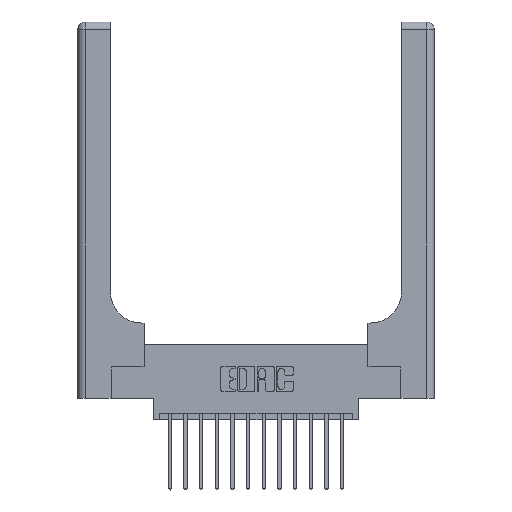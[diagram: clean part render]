
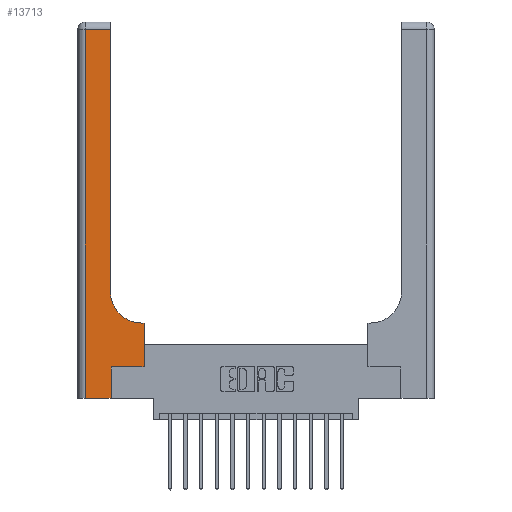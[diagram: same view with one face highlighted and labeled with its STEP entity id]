
A CAD part, top view. The second image highlights one B-rep face of the part: STEP entity #13713.
In plain terms, the highlighted planar face has unit normal (0, 0, 1).
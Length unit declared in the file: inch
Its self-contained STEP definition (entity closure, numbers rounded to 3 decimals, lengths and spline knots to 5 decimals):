
#178 = EDGE_LOOP ( 'NONE', ( #1392, #8823, #4868, #6654, #13039, #760, #14122, #10575, #12890 ) ) ;
#760 = ORIENTED_EDGE ( 'NONE', *, *, #14754, .T. ) ;
#984 = CARTESIAN_POINT ( 'NONE',  ( 0.06, 2.94, 0.37 ) ) ;
#1244 = DIRECTION ( 'NONE',  ( 0., 0., -1. ) ) ;
#1270 = DIRECTION ( 'NONE',  ( 1., 0., 0. ) ) ;
#1392 = ORIENTED_EDGE ( 'NONE', *, *, #10980, .T. ) ;
#1998 = EDGE_CURVE ( 'NONE', #4549, #11544, #16536, .T. ) ;
#2104 = LINE ( 'NONE', #8802, #8312 ) ;
#2680 = DIRECTION ( 'NONE',  ( 0., 0., -1. ) ) ;
#2692 = CARTESIAN_POINT ( 'NONE',  ( 0.26, 2.94, 0.37 ) ) ;
#3514 = EDGE_CURVE ( 'NONE', #14203, #12566, #5330, .T. ) ;
#3596 = VECTOR ( 'NONE', #9896, 39.37008 ) ;
#4549 = VERTEX_POINT ( 'NONE', #10410 ) ;
#4627 = VECTOR ( 'NONE', #4942, 39.37008 ) ;
#4661 = CIRCLE ( 'NONE', #5664, 0.25 ) ;
#4868 = ORIENTED_EDGE ( 'NONE', *, *, #14104, .T. ) ;
#4942 = DIRECTION ( 'NONE',  ( 0., -1., 0. ) ) ;
#5330 = LINE ( 'NONE', #16295, #11973 ) ;
#5664 = AXIS2_PLACEMENT_3D ( 'NONE', #9179, #1244, #10537 ) ;
#5874 = CARTESIAN_POINT ( 'NONE',  ( 0.528, 0.25, 0.37 ) ) ;
#6355 = EDGE_CURVE ( 'NONE', #7479, #15930, #13785, .T. ) ;
#6401 = VERTEX_POINT ( 'NONE', #9953 ) ;
#6654 = ORIENTED_EDGE ( 'NONE', *, *, #6355, .T. ) ;
#7205 = LINE ( 'NONE', #5874, #14267 ) ;
#7479 = VERTEX_POINT ( 'NONE', #8169 ) ;
#7926 = CARTESIAN_POINT ( 'NONE',  ( 0.265, 0., 0.37 ) ) ;
#7965 = CARTESIAN_POINT ( 'NONE',  ( 0., 3., 0.37 ) ) ;
#8169 = CARTESIAN_POINT ( 'NONE',  ( 0.06, 0., 0.37 ) ) ;
#8312 = VECTOR ( 'NONE', #16775, 39.37008 ) ;
#8544 = CARTESIAN_POINT ( 'NONE',  ( 0., 0., 0.37 ) ) ;
#8802 = CARTESIAN_POINT ( 'NONE',  ( 0.265, 0., 0.37 ) ) ;
#8823 = ORIENTED_EDGE ( 'NONE', *, *, #3514, .T. ) ;
#9179 = CARTESIAN_POINT ( 'NONE',  ( 0.51, 0.85, 0.37 ) ) ;
#9453 = VECTOR ( 'NONE', #14989, 39.37008 ) ;
#9690 = DIRECTION ( 'NONE',  ( -1., 0., 0. ) ) ;
#9896 = DIRECTION ( 'NONE',  ( 1., 0., 0. ) ) ;
#9953 = CARTESIAN_POINT ( 'NONE',  ( 0.265, 0.25, 0.37 ) ) ;
#10099 = VECTOR ( 'NONE', #12071, 39.37008 ) ;
#10410 = CARTESIAN_POINT ( 'NONE',  ( 0.528, 0.6, 0.37 ) ) ;
#10510 = LINE ( 'NONE', #10718, #10099 ) ;
#10537 = DIRECTION ( 'NONE',  ( 1., 0., 0. ) ) ;
#10575 = ORIENTED_EDGE ( 'NONE', *, *, #1998, .T. ) ;
#10616 = PLANE ( 'NONE',  #15116 ) ;
#10718 = CARTESIAN_POINT ( 'NONE',  ( 0.26, 3., 0.37 ) ) ;
#10980 = EDGE_CURVE ( 'NONE', #16078, #14203, #10510, .T. ) ;
#11180 = EDGE_CURVE ( 'NONE', #16935, #4549, #7205, .T. ) ;
#11438 = CARTESIAN_POINT ( 'NONE',  ( 0.528, 0.25, 0.37 ) ) ;
#11544 = VERTEX_POINT ( 'NONE', #14835 ) ;
#11868 = LINE ( 'NONE', #17193, #14990 ) ;
#11973 = VECTOR ( 'NONE', #9690, 39.37008 ) ;
#11975 = DIRECTION ( 'NONE',  ( -1., 0., 0. ) ) ;
#12071 = DIRECTION ( 'NONE',  ( 0., 1., 0. ) ) ;
#12566 = VERTEX_POINT ( 'NONE', #984 ) ;
#12890 = ORIENTED_EDGE ( 'NONE', *, *, #13169, .T. ) ;
#12904 = CARTESIAN_POINT ( 'NONE',  ( 0.06, 3., 0.37 ) ) ;
#13039 = ORIENTED_EDGE ( 'NONE', *, *, #15210, .T. ) ;
#13169 = EDGE_CURVE ( 'NONE', #11544, #16078, #4661, .T. ) ;
#13580 = FACE_OUTER_BOUND ( 'NONE', #178, .T. ) ;
#13619 = CARTESIAN_POINT ( 'NONE',  ( 0.26, 0.85, 0.37 ) ) ;
#13666 = CARTESIAN_POINT ( 'NONE',  ( 0.26, 0.6, 0.37 ) ) ;
#13713 = ADVANCED_FACE ( 'NONE', ( #13580 ), #10616, .F. ) ;
#13785 = LINE ( 'NONE', #8544, #3596 ) ;
#13878 = DIRECTION ( 'NONE',  ( 0., 1., 0. ) ) ;
#14104 = EDGE_CURVE ( 'NONE', #12566, #7479, #14810, .T. ) ;
#14122 = ORIENTED_EDGE ( 'NONE', *, *, #11180, .T. ) ;
#14203 = VERTEX_POINT ( 'NONE', #2692 ) ;
#14267 = VECTOR ( 'NONE', #13878, 39.37008 ) ;
#14754 = EDGE_CURVE ( 'NONE', #6401, #16935, #11868, .T. ) ;
#14810 = LINE ( 'NONE', #12904, #4627 ) ;
#14835 = CARTESIAN_POINT ( 'NONE',  ( 0.51, 0.6, 0.37 ) ) ;
#14989 = DIRECTION ( 'NONE',  ( -1., 0., 0. ) ) ;
#14990 = VECTOR ( 'NONE', #1270, 39.37008 ) ;
#15116 = AXIS2_PLACEMENT_3D ( 'NONE', #7965, #2680, #11975 ) ;
#15210 = EDGE_CURVE ( 'NONE', #15930, #6401, #2104, .T. ) ;
#15930 = VERTEX_POINT ( 'NONE', #7926 ) ;
#16078 = VERTEX_POINT ( 'NONE', #13619 ) ;
#16295 = CARTESIAN_POINT ( 'NONE',  ( 0., 2.94, 0.37 ) ) ;
#16536 = LINE ( 'NONE', #13666, #9453 ) ;
#16775 = DIRECTION ( 'NONE',  ( 0., 1., 0. ) ) ;
#16935 = VERTEX_POINT ( 'NONE', #11438 ) ;
#17193 = CARTESIAN_POINT ( 'NONE',  ( 0.265, 0.25, 0.37 ) ) ;
